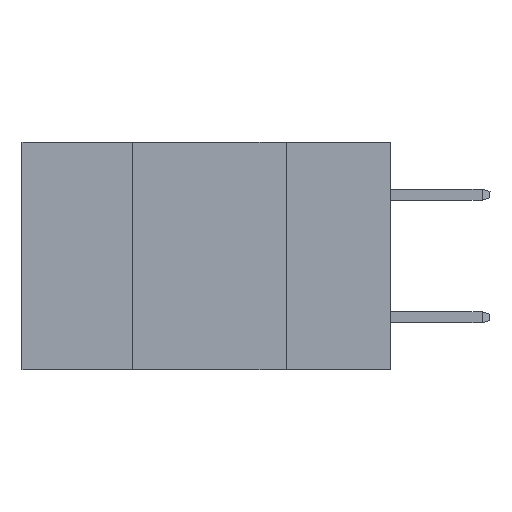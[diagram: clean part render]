
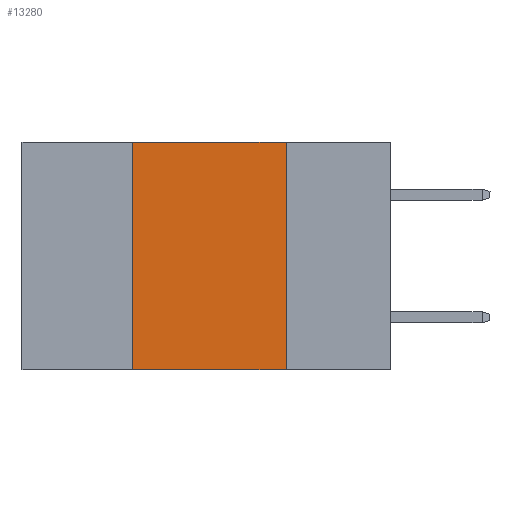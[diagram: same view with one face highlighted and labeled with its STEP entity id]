
A CAD part, left-side view. The second image highlights one B-rep face of the part: STEP entity #13280.
In plain terms, the highlighted planar face has unit normal (-1, 0, 0).
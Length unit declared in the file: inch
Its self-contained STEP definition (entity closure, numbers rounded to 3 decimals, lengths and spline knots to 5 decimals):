
#249 = ORIENTED_EDGE ( 'NONE', *, *, #1491, .F. ) ;
#1491 = EDGE_CURVE ( 'NONE', #12080, #10613, #12229, .T. ) ;
#1999 = CARTESIAN_POINT ( 'NONE',  ( 0., 0.6, 0. ) ) ;
#2012 = LINE ( 'NONE', #13225, #7361 ) ;
#2471 = ORIENTED_EDGE ( 'NONE', *, *, #3565, .F. ) ;
#2936 = VECTOR ( 'NONE', #11515, 39.37008 ) ;
#3106 = DIRECTION ( 'NONE',  ( 1., 0., 0. ) ) ;
#3304 = LINE ( 'NONE', #5296, #2936 ) ;
#3565 = EDGE_CURVE ( 'NONE', #10613, #10282, #2012, .T. ) ;
#3837 = ORIENTED_EDGE ( 'NONE', *, *, #12930, .F. ) ;
#4634 = CARTESIAN_POINT ( 'NONE',  ( 0., 0.17, 0. ) ) ;
#5036 = AXIS2_PLACEMENT_3D ( 'NONE', #1999, #3106, #10438 ) ;
#5040 = CARTESIAN_POINT ( 'NONE',  ( 0., 0.42, 0. ) ) ;
#5296 = CARTESIAN_POINT ( 'NONE',  ( 0., 0.6, -0.37 ) ) ;
#5383 = VERTEX_POINT ( 'NONE', #7708 ) ;
#5841 = VECTOR ( 'NONE', #12884, 39.37008 ) ;
#6982 = ORIENTED_EDGE ( 'NONE', *, *, #11599, .T. ) ;
#7361 = VECTOR ( 'NONE', #7770, 39.37008 ) ;
#7708 = CARTESIAN_POINT ( 'NONE',  ( 0., 0.42, -0.37 ) ) ;
#7770 = DIRECTION ( 'NONE',  ( 0., 0., -1. ) ) ;
#8365 = PLANE ( 'NONE',  #5036 ) ;
#9175 = VECTOR ( 'NONE', #13377, 39.37008 ) ;
#9249 = FACE_OUTER_BOUND ( 'NONE', #10953, .T. ) ;
#9822 = CARTESIAN_POINT ( 'NONE',  ( 0., 0.42, 0. ) ) ;
#10282 = VERTEX_POINT ( 'NONE', #13353 ) ;
#10438 = DIRECTION ( 'NONE',  ( 0., 0., -1. ) ) ;
#10613 = VERTEX_POINT ( 'NONE', #4634 ) ;
#10953 = EDGE_LOOP ( 'NONE', ( #2471, #249, #3837, #6982 ) ) ;
#11347 = LINE ( 'NONE', #9822, #5841 ) ;
#11515 = DIRECTION ( 'NONE',  ( 0., -1., 0. ) ) ;
#11599 = EDGE_CURVE ( 'NONE', #5383, #10282, #3304, .T. ) ;
#12080 = VERTEX_POINT ( 'NONE', #5040 ) ;
#12229 = LINE ( 'NONE', #13114, #9175 ) ;
#12884 = DIRECTION ( 'NONE',  ( 0., 0., 1. ) ) ;
#12930 = EDGE_CURVE ( 'NONE', #5383, #12080, #11347, .T. ) ;
#13114 = CARTESIAN_POINT ( 'NONE',  ( 0., 0.6, 0. ) ) ;
#13225 = CARTESIAN_POINT ( 'NONE',  ( 0., 0.17, 0. ) ) ;
#13280 = ADVANCED_FACE ( 'NONE', ( #9249 ), #8365, .F. ) ;
#13353 = CARTESIAN_POINT ( 'NONE',  ( 0., 0.17, -0.37 ) ) ;
#13377 = DIRECTION ( 'NONE',  ( 0., -1., 0. ) ) ;
